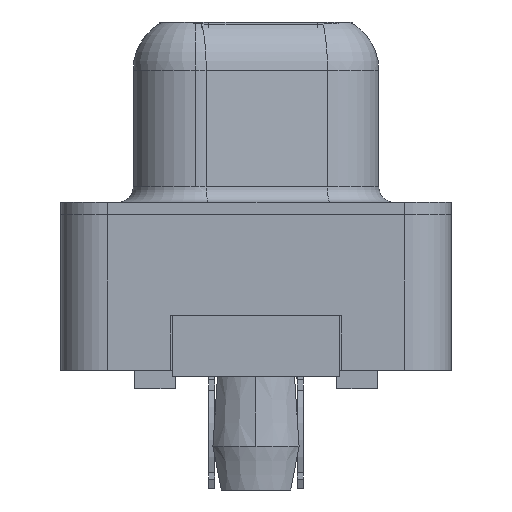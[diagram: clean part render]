
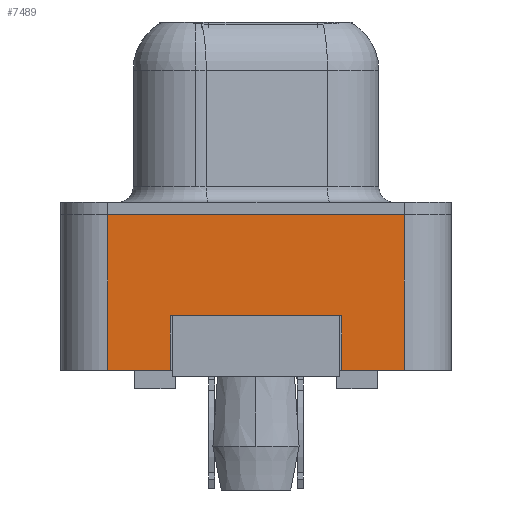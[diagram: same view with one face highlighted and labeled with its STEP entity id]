
A CAD part, left-side view. The second image highlights one B-rep face of the part: STEP entity #7489.
In plain terms, the highlighted planar face has unit normal (-1, 0, 0).
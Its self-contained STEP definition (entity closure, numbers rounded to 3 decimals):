
#415 = CARTESIAN_POINT ( 'NONE',  ( -2.945, 2.75, -3.25 ) ) ;
#712 = DIRECTION ( 'NONE',  ( 0., 0., 1. ) ) ;
#776 = EDGE_CURVE ( 'NONE', #4435, #18501, #5030, .T. ) ;
#793 = VERTEX_POINT ( 'NONE', #10798 ) ;
#875 = EDGE_CURVE ( 'NONE', #1440, #793, #18075, .T. ) ;
#1159 = ORIENTED_EDGE ( 'NONE', *, *, #4103, .T. ) ;
#1244 = CARTESIAN_POINT ( 'NONE',  ( -2.945, -4.775, -5. ) ) ;
#1268 = VERTEX_POINT ( 'NONE', #3663 ) ;
#1269 = CARTESIAN_POINT ( 'NONE',  ( -2.945, 4.775, -5. ) ) ;
#1440 = VERTEX_POINT ( 'NONE', #11151 ) ;
#1445 = AXIS2_PLACEMENT_3D ( 'NONE', #2103, #13642, #712 ) ;
#1631 = VECTOR ( 'NONE', #11008, 1000. ) ;
#1643 = VERTEX_POINT ( 'NONE', #13397 ) ;
#2103 = CARTESIAN_POINT ( 'NONE',  ( -2.945, -4.775, -5. ) ) ;
#2576 = LINE ( 'NONE', #1269, #5437 ) ;
#2890 = CARTESIAN_POINT ( 'NONE',  ( -2.945, -4.775, -5. ) ) ;
#3513 = VECTOR ( 'NONE', #7643, 1000. ) ;
#3663 = CARTESIAN_POINT ( 'NONE',  ( -2.945, 4.775, -5. ) ) ;
#4103 = EDGE_CURVE ( 'NONE', #1268, #793, #4930, .T. ) ;
#4435 = VERTEX_POINT ( 'NONE', #10499 ) ;
#4930 = LINE ( 'NONE', #17875, #17818 ) ;
#5030 = LINE ( 'NONE', #13441, #11190 ) ;
#5086 = ORIENTED_EDGE ( 'NONE', *, *, #776, .T. ) ;
#5120 = CARTESIAN_POINT ( 'NONE',  ( -2.945, 2.75, -3.25 ) ) ;
#5208 = ORIENTED_EDGE ( 'NONE', *, *, #5850, .T. ) ;
#5437 = VECTOR ( 'NONE', #16671, 1000. ) ;
#5674 = ORIENTED_EDGE ( 'NONE', *, *, #8862, .T. ) ;
#5681 = LINE ( 'NONE', #1244, #18077 ) ;
#5850 = EDGE_CURVE ( 'NONE', #18501, #7852, #12065, .T. ) ;
#6139 = VERTEX_POINT ( 'NONE', #13985 ) ;
#7489 = ADVANCED_FACE ( 'NONE', ( #14962 ), #15051, .T. ) ;
#7643 = DIRECTION ( 'NONE',  ( 0., -1., 0. ) ) ;
#7852 = VERTEX_POINT ( 'NONE', #2890 ) ;
#8547 = LINE ( 'NONE', #415, #10198 ) ;
#8862 = EDGE_CURVE ( 'NONE', #7852, #6139, #5681, .T. ) ;
#9204 = DIRECTION ( 'NONE',  ( 0., 0., -1. ) ) ;
#9747 = EDGE_LOOP ( 'NONE', ( #5086, #5208, #5674, #18682, #12134, #1159, #12369, #17756 ) ) ;
#10198 = VECTOR ( 'NONE', #17602, 1000. ) ;
#10221 = EDGE_CURVE ( 'NONE', #1268, #1643, #2576, .T. ) ;
#10478 = EDGE_CURVE ( 'NONE', #4435, #1440, #8547, .T. ) ;
#10499 = CARTESIAN_POINT ( 'NONE',  ( -2.945, -2.75, -3.25 ) ) ;
#10798 = CARTESIAN_POINT ( 'NONE',  ( -2.945, 2.75, -5. ) ) ;
#10888 = DIRECTION ( 'NONE',  ( 0., 0., -1. ) ) ;
#10964 = DIRECTION ( 'NONE',  ( 0., -1., 0. ) ) ;
#11008 = DIRECTION ( 'NONE',  ( 0., -1., 0. ) ) ;
#11151 = CARTESIAN_POINT ( 'NONE',  ( -2.945, 2.75, -3.25 ) ) ;
#11190 = VECTOR ( 'NONE', #9204, 1000. ) ;
#11874 = CARTESIAN_POINT ( 'NONE',  ( -2.945, -4.775, -5. ) ) ;
#12065 = LINE ( 'NONE', #11874, #3513 ) ;
#12134 = ORIENTED_EDGE ( 'NONE', *, *, #10221, .F. ) ;
#12369 = ORIENTED_EDGE ( 'NONE', *, *, #875, .F. ) ;
#13008 = VECTOR ( 'NONE', #10888, 1000. ) ;
#13397 = CARTESIAN_POINT ( 'NONE',  ( -2.945, 4.775, 0. ) ) ;
#13441 = CARTESIAN_POINT ( 'NONE',  ( -2.945, -2.75, -3.25 ) ) ;
#13642 = DIRECTION ( 'NONE',  ( -1., 0., 0. ) ) ;
#13841 = LINE ( 'NONE', #15071, #1631 ) ;
#13985 = CARTESIAN_POINT ( 'NONE',  ( -2.945, -4.775, 0. ) ) ;
#14360 = CARTESIAN_POINT ( 'NONE',  ( -2.945, -2.75, -5. ) ) ;
#14962 = FACE_OUTER_BOUND ( 'NONE', #9747, .T. ) ;
#15051 = PLANE ( 'NONE',  #1445 ) ;
#15071 = CARTESIAN_POINT ( 'NONE',  ( -2.945, -4.775, 0. ) ) ;
#15874 = DIRECTION ( 'NONE',  ( 0., 0., 1. ) ) ;
#16671 = DIRECTION ( 'NONE',  ( 0., 0., 1. ) ) ;
#17602 = DIRECTION ( 'NONE',  ( 0., 1., 0. ) ) ;
#17756 = ORIENTED_EDGE ( 'NONE', *, *, #10478, .F. ) ;
#17818 = VECTOR ( 'NONE', #10964, 1000. ) ;
#17875 = CARTESIAN_POINT ( 'NONE',  ( -2.945, -4.775, -5. ) ) ;
#17900 = EDGE_CURVE ( 'NONE', #1643, #6139, #13841, .T. ) ;
#18075 = LINE ( 'NONE', #5120, #13008 ) ;
#18077 = VECTOR ( 'NONE', #15874, 1000. ) ;
#18501 = VERTEX_POINT ( 'NONE', #14360 ) ;
#18682 = ORIENTED_EDGE ( 'NONE', *, *, #17900, .F. ) ;
